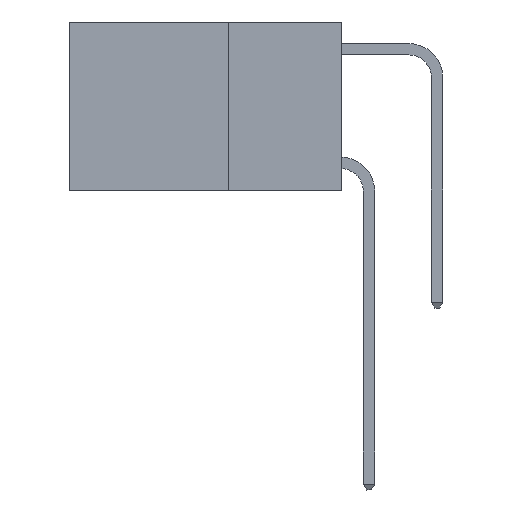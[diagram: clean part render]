
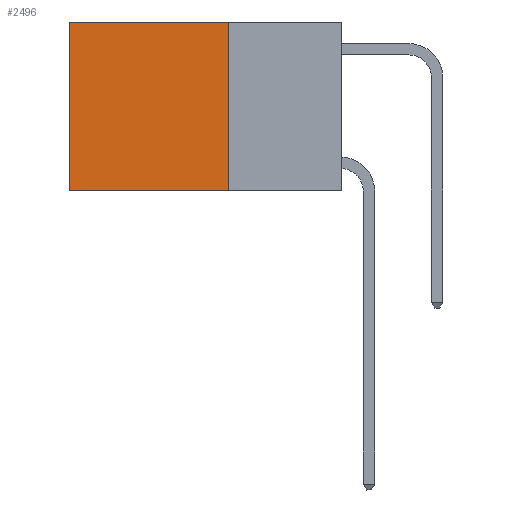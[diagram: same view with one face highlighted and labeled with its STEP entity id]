
A CAD part, left-side view. The second image highlights one B-rep face of the part: STEP entity #2496.
In plain terms, the highlighted planar face has unit normal (-1, 0, 0).
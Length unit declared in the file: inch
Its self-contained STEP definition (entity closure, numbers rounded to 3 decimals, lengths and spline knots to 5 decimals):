
#46 = EDGE_CURVE ( 'NONE', #2862, #4816, #6848, .T. ) ;
#391 = DIRECTION ( 'NONE',  ( 0., 0., -1. ) ) ;
#464 = CARTESIAN_POINT ( 'NONE',  ( 0.2625, 0.25, 0. ) ) ;
#780 = EDGE_CURVE ( 'NONE', #3480, #4816, #1053, .T. ) ;
#822 = EDGE_CURVE ( 'NONE', #3892, #3480, #7451, .T. ) ;
#1053 = LINE ( 'NONE', #3772, #6015 ) ;
#1340 = ORIENTED_EDGE ( 'NONE', *, *, #822, .F. ) ;
#1758 = AXIS2_PLACEMENT_3D ( 'NONE', #464, #10640, #5802 ) ;
#2117 = CARTESIAN_POINT ( 'NONE',  ( 0.2625, 0.6, 0. ) ) ;
#2451 = ORIENTED_EDGE ( 'NONE', *, *, #46, .T. ) ;
#2496 = ADVANCED_FACE ( 'NONE', ( #7550 ), #3126, .F. ) ;
#2508 = DIRECTION ( 'NONE',  ( 0., 1., 0. ) ) ;
#2638 = EDGE_LOOP ( 'NONE', ( #2451, #3988, #1340, #6687 ) ) ;
#2862 = VERTEX_POINT ( 'NONE', #2117 ) ;
#3126 = PLANE ( 'NONE',  #1758 ) ;
#3141 = EDGE_CURVE ( 'NONE', #3892, #2862, #10764, .T. ) ;
#3476 = CARTESIAN_POINT ( 'NONE',  ( 0.2625, 0.25, 0. ) ) ;
#3480 = VERTEX_POINT ( 'NONE', #9067 ) ;
#3699 = DIRECTION ( 'NONE',  ( 0., 0., -1. ) ) ;
#3772 = CARTESIAN_POINT ( 'NONE',  ( 0.2625, 0.25, -0.37 ) ) ;
#3892 = VERTEX_POINT ( 'NONE', #8771 ) ;
#3988 = ORIENTED_EDGE ( 'NONE', *, *, #780, .F. ) ;
#4625 = CARTESIAN_POINT ( 'NONE',  ( 0.2625, 0.6, 0. ) ) ;
#4816 = VERTEX_POINT ( 'NONE', #9066 ) ;
#5802 = DIRECTION ( 'NONE',  ( 0., 0., -1. ) ) ;
#6015 = VECTOR ( 'NONE', #2508, 39.37008 ) ;
#6687 = ORIENTED_EDGE ( 'NONE', *, *, #3141, .T. ) ;
#6848 = LINE ( 'NONE', #4625, #7112 ) ;
#7112 = VECTOR ( 'NONE', #3699, 39.37008 ) ;
#7203 = VECTOR ( 'NONE', #391, 39.37008 ) ;
#7451 = LINE ( 'NONE', #8435, #7203 ) ;
#7550 = FACE_OUTER_BOUND ( 'NONE', #2638, .T. ) ;
#8435 = CARTESIAN_POINT ( 'NONE',  ( 0.2625, 0.25, 0. ) ) ;
#8691 = VECTOR ( 'NONE', #9395, 39.37008 ) ;
#8771 = CARTESIAN_POINT ( 'NONE',  ( 0.2625, 0.25, 0. ) ) ;
#9066 = CARTESIAN_POINT ( 'NONE',  ( 0.2625, 0.6, -0.37 ) ) ;
#9067 = CARTESIAN_POINT ( 'NONE',  ( 0.2625, 0.25, -0.37 ) ) ;
#9395 = DIRECTION ( 'NONE',  ( 0., 1., 0. ) ) ;
#10640 = DIRECTION ( 'NONE',  ( 1., 0., 0. ) ) ;
#10764 = LINE ( 'NONE', #3476, #8691 ) ;
